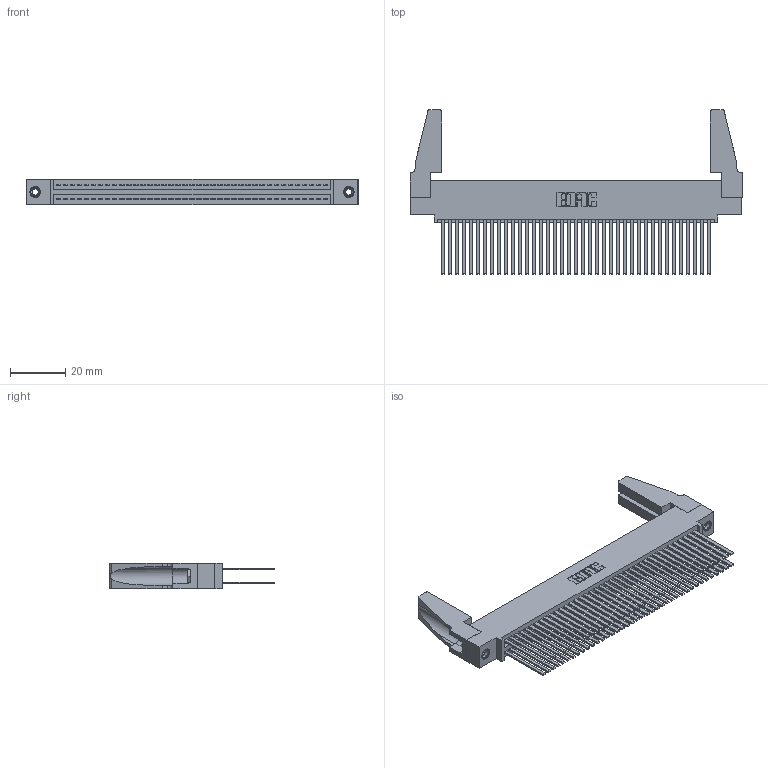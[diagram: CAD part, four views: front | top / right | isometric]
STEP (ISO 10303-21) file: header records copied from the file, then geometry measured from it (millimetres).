
FILE_DESCRIPTION (( 'STEP AP203' ), '1' );
FILE_NAME ('345-078-544-588.STEP', '2019-10-31T16:21:37', ( '' ), ( '' ), 'SwSTEP 2.0', 'SolidWorks 2016', '' );
FILE_SCHEMA (( 'CONFIG_CONTROL_DESIGN' ));
Length unit declared in the file: inch
Products named in the file (5): 345-292-001_345-293-144; 345-078-544-588; 345 Part_0.110 Offset - 0.156 Dia-TH; 345-250-001_345-250-001-102; 345-220-078_345-220-088
Assembly tree (83 placements, depth 2):
  345-078-544-588
    345 Part_0.110 Offset - 0.156 Dia-TH
    345-292-001_345-293-144  x78
    345-250-001_345-250-001-102  x2
    345-220-078_345-220-088  x2
Bounding box: 120.29 x 59.61 x 9.4 mm (x, y, z)
Volume: 15930.2 mm3; surface area: 25101.4 mm2
Topology: 83 solids, 83 shells, 3686 faces, 10885 edges, 7142 vertices
Faces by surface type: plane 2418, cylinder 1252, cone 12, torus 4
Entity records: 33100 total; most frequent: CARTESIAN_POINT 5546, ORIENTED_EDGE 5440, DIRECTION 4896, EDGE_CURVE 2720, VECTOR 2394, LINE 2394, VERTEX_POINT 1806, AXIS2_PLACEMENT_3D 1251
